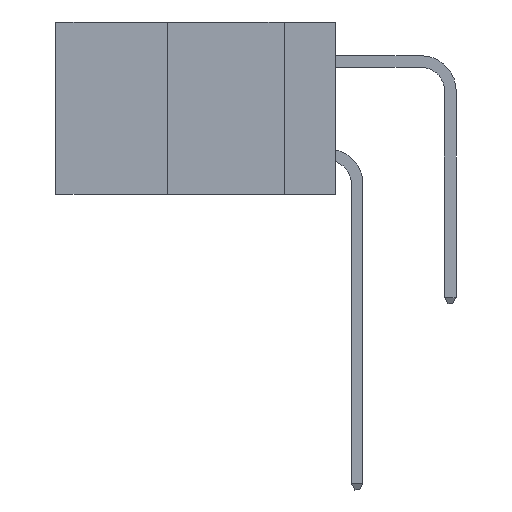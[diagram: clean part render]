
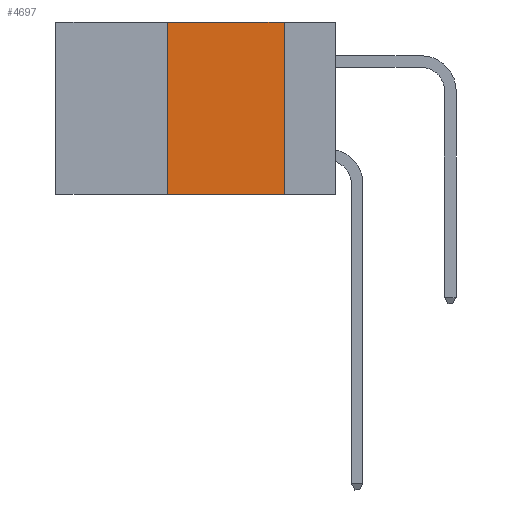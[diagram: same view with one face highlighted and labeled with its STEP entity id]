
A CAD part, left-side view. The second image highlights one B-rep face of the part: STEP entity #4697.
In plain terms, the highlighted planar face has unit normal (-1, 0, 0).
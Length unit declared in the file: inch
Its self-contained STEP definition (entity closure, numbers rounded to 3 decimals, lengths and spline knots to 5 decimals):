
#75 = AXIS2_PLACEMENT_3D ( 'NONE', #4662, #6798, #16132 ) ;
#1364 = VERTEX_POINT ( 'NONE', #8970 ) ;
#1557 = DIRECTION ( 'NONE',  ( 0., -1., 0. ) ) ;
#3113 = VERTEX_POINT ( 'NONE', #22083 ) ;
#3546 = CARTESIAN_POINT ( 'NONE',  ( 0., 0.36, -0.37 ) ) ;
#3738 = DIRECTION ( 'NONE',  ( 0., 0., -1. ) ) ;
#4112 = ORIENTED_EDGE ( 'NONE', *, *, #8807, .F. ) ;
#4662 = CARTESIAN_POINT ( 'NONE',  ( 0., 0.6, 0. ) ) ;
#4697 = ADVANCED_FACE ( 'NONE', ( #6064 ), #18966, .F. ) ;
#4737 = ORIENTED_EDGE ( 'NONE', *, *, #17766, .F. ) ;
#5814 = ORIENTED_EDGE ( 'NONE', *, *, #11379, .T. ) ;
#5899 = VECTOR ( 'NONE', #18567, 39.37008 ) ;
#6064 = FACE_OUTER_BOUND ( 'NONE', #8193, .T. ) ;
#6798 = DIRECTION ( 'NONE',  ( 1., 0., 0. ) ) ;
#8003 = LINE ( 'NONE', #12482, #11363 ) ;
#8193 = EDGE_LOOP ( 'NONE', ( #4737, #4112, #18497, #5814 ) ) ;
#8699 = VECTOR ( 'NONE', #1557, 39.37008 ) ;
#8807 = EDGE_CURVE ( 'NONE', #3113, #23444, #22860, .T. ) ;
#8970 = CARTESIAN_POINT ( 'NONE',  ( 0., 0.11, -0.37 ) ) ;
#9026 = CARTESIAN_POINT ( 'NONE',  ( 0., 0.36, 0. ) ) ;
#10898 = LINE ( 'NONE', #9026, #27166 ) ;
#11363 = VECTOR ( 'NONE', #3738, 39.37008 ) ;
#11379 = EDGE_CURVE ( 'NONE', #22987, #1364, #12050, .T. ) ;
#12050 = LINE ( 'NONE', #27252, #8699 ) ;
#12482 = CARTESIAN_POINT ( 'NONE',  ( 0., 0.11, 0. ) ) ;
#16132 = DIRECTION ( 'NONE',  ( 0., 0., -1. ) ) ;
#17766 = EDGE_CURVE ( 'NONE', #23444, #1364, #8003, .T. ) ;
#18497 = ORIENTED_EDGE ( 'NONE', *, *, #25709, .F. ) ;
#18567 = DIRECTION ( 'NONE',  ( 0., -1., 0. ) ) ;
#18966 = PLANE ( 'NONE',  #75 ) ;
#19611 = DIRECTION ( 'NONE',  ( 0., 0., 1. ) ) ;
#22083 = CARTESIAN_POINT ( 'NONE',  ( 0., 0.36, 0. ) ) ;
#22787 = CARTESIAN_POINT ( 'NONE',  ( 0., 0.6, 0. ) ) ;
#22860 = LINE ( 'NONE', #22787, #5899 ) ;
#22987 = VERTEX_POINT ( 'NONE', #3546 ) ;
#23444 = VERTEX_POINT ( 'NONE', #24434 ) ;
#24434 = CARTESIAN_POINT ( 'NONE',  ( 0., 0.11, 0. ) ) ;
#25709 = EDGE_CURVE ( 'NONE', #22987, #3113, #10898, .T. ) ;
#27166 = VECTOR ( 'NONE', #19611, 39.37008 ) ;
#27252 = CARTESIAN_POINT ( 'NONE',  ( 0., 0.6, -0.37 ) ) ;
